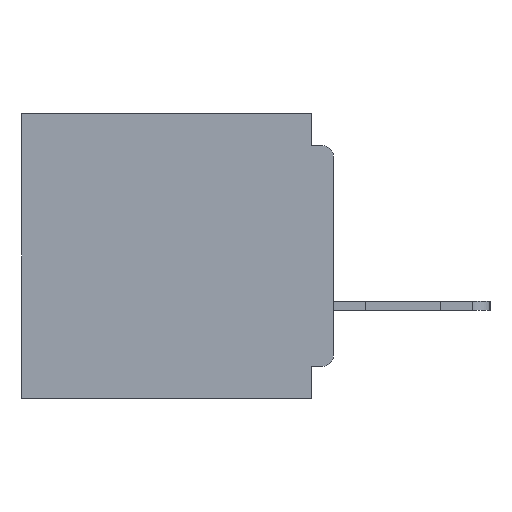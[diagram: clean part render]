
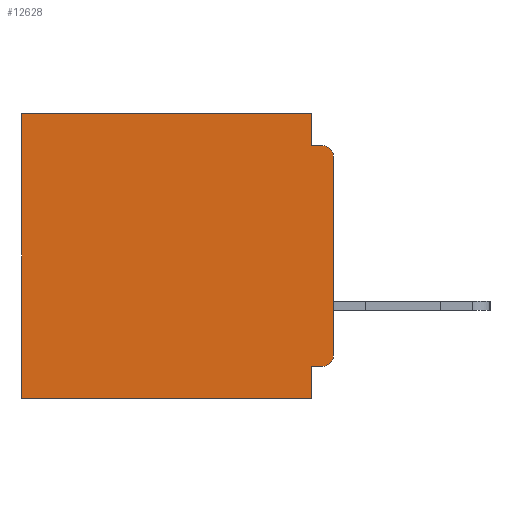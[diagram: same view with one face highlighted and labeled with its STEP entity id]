
A CAD part, left-side view. The second image highlights one B-rep face of the part: STEP entity #12628.
In plain terms, the highlighted planar face has unit normal (-1, 0, 0).
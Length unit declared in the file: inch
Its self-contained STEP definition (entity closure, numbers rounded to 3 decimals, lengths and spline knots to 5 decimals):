
#323 = VERTEX_POINT ( 'NONE', #51474 ) ;
#1076 = LINE ( 'NONE', #30662, #30873 ) ;
#1642 = LINE ( 'NONE', #3110, #18093 ) ;
#3110 = CARTESIAN_POINT ( 'NONE',  ( 0.3, 0.031, 0. ) ) ;
#3112 = CARTESIAN_POINT ( 'NONE',  ( 0.3, 0.437, 0. ) ) ;
#3224 = LINE ( 'NONE', #5388, #34228 ) ;
#3475 = CARTESIAN_POINT ( 'NONE',  ( 0.3, 0., -0.4 ) ) ;
#4136 = VERTEX_POINT ( 'NONE', #39873 ) ;
#4367 = EDGE_CURVE ( 'NONE', #323, #42545, #46361, .T. ) ;
#4395 = ORIENTED_EDGE ( 'NONE', *, *, #49945, .F. ) ;
#5388 = CARTESIAN_POINT ( 'NONE',  ( 0.3, 0., -0.355 ) ) ;
#5394 = VERTEX_POINT ( 'NONE', #51949 ) ;
#5737 = LINE ( 'NONE', #34325, #16521 ) ;
#6252 = LINE ( 'NONE', #28744, #27841 ) ;
#8021 = ORIENTED_EDGE ( 'NONE', *, *, #4367, .T. ) ;
#8555 = DIRECTION ( 'NONE',  ( 0., 0., -1. ) ) ;
#8789 = CARTESIAN_POINT ( 'NONE',  ( 0.3, 0.031, -0.045 ) ) ;
#9511 = VECTOR ( 'NONE', #16584, 39.37008 ) ;
#9589 = CARTESIAN_POINT ( 'NONE',  ( 0.3, 0.015, -0.06 ) ) ;
#10284 = DIRECTION ( 'NONE',  ( 0., 1., 0. ) ) ;
#11612 = DIRECTION ( 'NONE',  ( 0., 0., -1. ) ) ;
#11743 = ORIENTED_EDGE ( 'NONE', *, *, #12140, .F. ) ;
#12140 = EDGE_CURVE ( 'NONE', #4136, #45876, #1642, .T. ) ;
#12493 = EDGE_CURVE ( 'NONE', #29604, #25216, #21885, .T. ) ;
#12513 = CARTESIAN_POINT ( 'NONE',  ( 0.3, 0., -0.045 ) ) ;
#12628 = ADVANCED_FACE ( 'NONE', ( #15504 ), #42792, .F. ) ;
#13462 = CARTESIAN_POINT ( 'NONE',  ( 0.3, 0.031, -0.355 ) ) ;
#13657 = DIRECTION ( 'NONE',  ( 0., 0., -1. ) ) ;
#14130 = EDGE_LOOP ( 'NONE', ( #41520, #37036, #23038, #11743, #21878, #35714, #4395, #20502, #15740, #8021 ) ) ;
#14531 = CARTESIAN_POINT ( 'NONE',  ( 0.3, 0., -0.4 ) ) ;
#15056 = VERTEX_POINT ( 'NONE', #40761 ) ;
#15504 = FACE_OUTER_BOUND ( 'NONE', #14130, .T. ) ;
#15740 = ORIENTED_EDGE ( 'NONE', *, *, #26115, .F. ) ;
#16521 = VECTOR ( 'NONE', #26234, 39.37008 ) ;
#16584 = DIRECTION ( 'NONE',  ( 0., -1., 0. ) ) ;
#17180 = DIRECTION ( 'NONE',  ( -1., 0., 0. ) ) ;
#18093 = VECTOR ( 'NONE', #31435, 39.37008 ) ;
#18111 = VERTEX_POINT ( 'NONE', #13462 ) ;
#18198 = AXIS2_PLACEMENT_3D ( 'NONE', #9589, #37880, #13657 ) ;
#18606 = DIRECTION ( 'NONE',  ( 1., 0., 0. ) ) ;
#18917 = CARTESIAN_POINT ( 'NONE',  ( 0.3, 0., 0. ) ) ;
#19683 = EDGE_CURVE ( 'NONE', #29604, #42545, #41489, .T. ) ;
#20049 = VECTOR ( 'NONE', #11612, 39.37008 ) ;
#20051 = CARTESIAN_POINT ( 'NONE',  ( 0.3, 0.015, -0.045 ) ) ;
#20502 = ORIENTED_EDGE ( 'NONE', *, *, #48280, .F. ) ;
#21878 = ORIENTED_EDGE ( 'NONE', *, *, #35597, .T. ) ;
#21885 = CIRCLE ( 'NONE', #18198, 0.015 ) ;
#23038 = ORIENTED_EDGE ( 'NONE', *, *, #47671, .F. ) ;
#23203 = EDGE_CURVE ( 'NONE', #38767, #5394, #5737, .T. ) ;
#25216 = VERTEX_POINT ( 'NONE', #20051 ) ;
#26115 = EDGE_CURVE ( 'NONE', #323, #18111, #3224, .T. ) ;
#26234 = DIRECTION ( 'NONE',  ( 0., 0., -1. ) ) ;
#27018 = CARTESIAN_POINT ( 'NONE',  ( 0.3, 0., -0.06 ) ) ;
#27841 = VECTOR ( 'NONE', #8555, 39.37008 ) ;
#28744 = CARTESIAN_POINT ( 'NONE',  ( 0.3, 0.031, -0.4 ) ) ;
#29604 = VERTEX_POINT ( 'NONE', #27018 ) ;
#30419 = VECTOR ( 'NONE', #39056, 39.37008 ) ;
#30662 = CARTESIAN_POINT ( 'NONE',  ( 0.3, 0., -0.4 ) ) ;
#30873 = VECTOR ( 'NONE', #10284, 39.37008 ) ;
#31435 = DIRECTION ( 'NONE',  ( 0., 0., -1. ) ) ;
#34228 = VECTOR ( 'NONE', #45812, 39.37008 ) ;
#34325 = CARTESIAN_POINT ( 'NONE',  ( 0.3, 0.437, -0.4 ) ) ;
#35597 = EDGE_CURVE ( 'NONE', #4136, #38767, #51772, .T. ) ;
#35714 = ORIENTED_EDGE ( 'NONE', *, *, #23203, .T. ) ;
#36739 = LINE ( 'NONE', #12513, #9511 ) ;
#36822 = CARTESIAN_POINT ( 'NONE',  ( 0.3, 0., -0.34 ) ) ;
#37036 = ORIENTED_EDGE ( 'NONE', *, *, #12493, .T. ) ;
#37880 = DIRECTION ( 'NONE',  ( -1., 0., 0. ) ) ;
#38767 = VERTEX_POINT ( 'NONE', #3112 ) ;
#39056 = DIRECTION ( 'NONE',  ( 0., 1., 0. ) ) ;
#39873 = CARTESIAN_POINT ( 'NONE',  ( 0.3, 0.031, 0. ) ) ;
#40761 = CARTESIAN_POINT ( 'NONE',  ( 0.3, 0.031, -0.4 ) ) ;
#41389 = CARTESIAN_POINT ( 'NONE',  ( 0.3, 0.015, -0.34 ) ) ;
#41489 = LINE ( 'NONE', #3475, #20049 ) ;
#41520 = ORIENTED_EDGE ( 'NONE', *, *, #19683, .F. ) ;
#42545 = VERTEX_POINT ( 'NONE', #36822 ) ;
#42792 = PLANE ( 'NONE',  #50610 ) ;
#43961 = AXIS2_PLACEMENT_3D ( 'NONE', #41389, #17180, #45399 ) ;
#45399 = DIRECTION ( 'NONE',  ( 0., 0., -1. ) ) ;
#45812 = DIRECTION ( 'NONE',  ( 0., 1., 0. ) ) ;
#45876 = VERTEX_POINT ( 'NONE', #8789 ) ;
#46361 = CIRCLE ( 'NONE', #43961, 0.015 ) ;
#46799 = DIRECTION ( 'NONE',  ( 0., 0., -1. ) ) ;
#47671 = EDGE_CURVE ( 'NONE', #45876, #25216, #36739, .T. ) ;
#48280 = EDGE_CURVE ( 'NONE', #18111, #15056, #6252, .T. ) ;
#49945 = EDGE_CURVE ( 'NONE', #15056, #5394, #1076, .T. ) ;
#50610 = AXIS2_PLACEMENT_3D ( 'NONE', #14531, #18606, #46799 ) ;
#51474 = CARTESIAN_POINT ( 'NONE',  ( 0.3, 0.015, -0.355 ) ) ;
#51772 = LINE ( 'NONE', #18917, #30419 ) ;
#51949 = CARTESIAN_POINT ( 'NONE',  ( 0.3, 0.437, -0.4 ) ) ;
